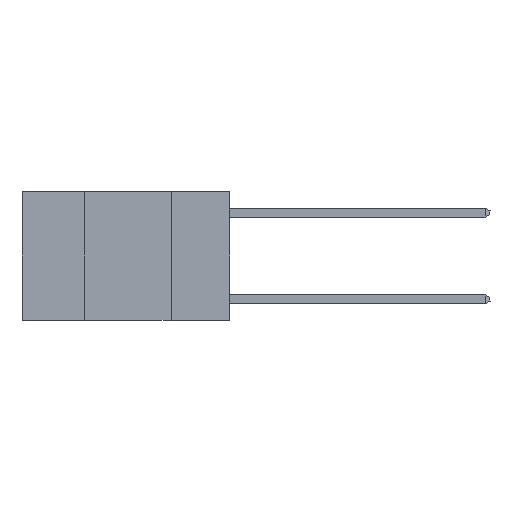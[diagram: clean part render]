
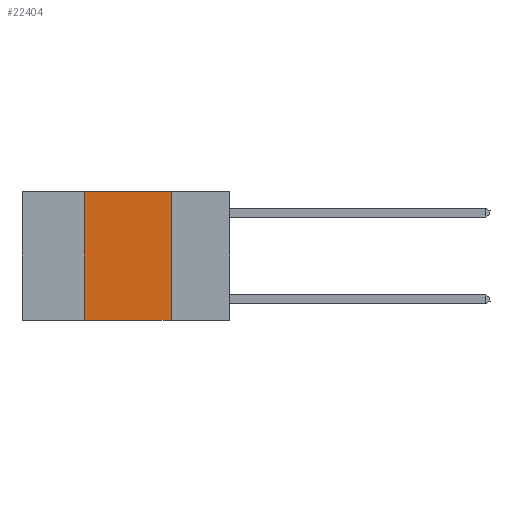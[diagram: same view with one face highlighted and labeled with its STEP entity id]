
A CAD part, left-side view. The second image highlights one B-rep face of the part: STEP entity #22404.
In plain terms, the highlighted planar face has unit normal (-1, 0, 0).
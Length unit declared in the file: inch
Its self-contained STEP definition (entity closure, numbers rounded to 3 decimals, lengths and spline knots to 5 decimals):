
#691 = CARTESIAN_POINT ( 'NONE',  ( 0., 0.6, 0. ) ) ;
#1932 = DIRECTION ( 'NONE',  ( 1., 0., 0. ) ) ;
#2383 = VECTOR ( 'NONE', #18991, 39.37008 ) ;
#3076 = CARTESIAN_POINT ( 'NONE',  ( 0., 0.17, 0. ) ) ;
#3793 = ORIENTED_EDGE ( 'NONE', *, *, #13794, .T. ) ;
#4104 = AXIS2_PLACEMENT_3D ( 'NONE', #19179, #1932, #11969 ) ;
#4429 = FACE_OUTER_BOUND ( 'NONE', #5923, .T. ) ;
#4853 = ORIENTED_EDGE ( 'NONE', *, *, #22548, .F. ) ;
#5877 = DIRECTION ( 'NONE',  ( 0., 0., -1. ) ) ;
#5923 = EDGE_LOOP ( 'NONE', ( #14179, #4853, #10479, #3793 ) ) ;
#8280 = LINE ( 'NONE', #691, #13982 ) ;
#8497 = CARTESIAN_POINT ( 'NONE',  ( 0., 0.42, 0. ) ) ;
#8531 = VERTEX_POINT ( 'NONE', #12908 ) ;
#9182 = PLANE ( 'NONE',  #4104 ) ;
#9586 = VECTOR ( 'NONE', #5877, 39.37008 ) ;
#10202 = CARTESIAN_POINT ( 'NONE',  ( 0., 0.17, 0. ) ) ;
#10479 = ORIENTED_EDGE ( 'NONE', *, *, #20072, .F. ) ;
#11969 = DIRECTION ( 'NONE',  ( 0., 0., -1. ) ) ;
#12908 = CARTESIAN_POINT ( 'NONE',  ( 0., 0.42, 0. ) ) ;
#13360 = DIRECTION ( 'NONE',  ( 0., -1., 0. ) ) ;
#13794 = EDGE_CURVE ( 'NONE', #21667, #31064, #21391, .T. ) ;
#13982 = VECTOR ( 'NONE', #20745, 39.37008 ) ;
#14179 = ORIENTED_EDGE ( 'NONE', *, *, #14672, .F. ) ;
#14672 = EDGE_CURVE ( 'NONE', #30554, #31064, #21307, .T. ) ;
#18991 = DIRECTION ( 'NONE',  ( 0., 0., 1. ) ) ;
#19179 = CARTESIAN_POINT ( 'NONE',  ( 0., 0.6, 0. ) ) ;
#20072 = EDGE_CURVE ( 'NONE', #21667, #8531, #23403, .T. ) ;
#20745 = DIRECTION ( 'NONE',  ( 0., -1., 0. ) ) ;
#21050 = VECTOR ( 'NONE', #13360, 39.37008 ) ;
#21307 = LINE ( 'NONE', #3076, #9586 ) ;
#21391 = LINE ( 'NONE', #28253, #21050 ) ;
#21667 = VERTEX_POINT ( 'NONE', #24225 ) ;
#22404 = ADVANCED_FACE ( 'NONE', ( #4429 ), #9182, .F. ) ;
#22548 = EDGE_CURVE ( 'NONE', #8531, #30554, #8280, .T. ) ;
#23403 = LINE ( 'NONE', #8497, #2383 ) ;
#23583 = CARTESIAN_POINT ( 'NONE',  ( 0., 0.17, -0.37 ) ) ;
#24225 = CARTESIAN_POINT ( 'NONE',  ( 0., 0.42, -0.37 ) ) ;
#28253 = CARTESIAN_POINT ( 'NONE',  ( 0., 0.6, -0.37 ) ) ;
#30554 = VERTEX_POINT ( 'NONE', #10202 ) ;
#31064 = VERTEX_POINT ( 'NONE', #23583 ) ;
